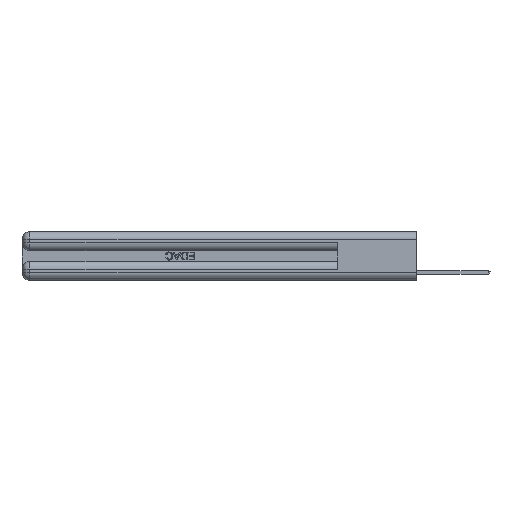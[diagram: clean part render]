
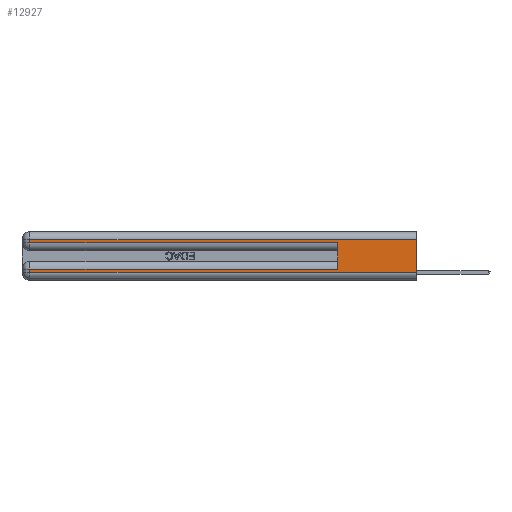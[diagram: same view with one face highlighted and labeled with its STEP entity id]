
A CAD part, left-side view. The second image highlights one B-rep face of the part: STEP entity #12927.
In plain terms, the highlighted planar face has unit normal (-1, 0, 0).
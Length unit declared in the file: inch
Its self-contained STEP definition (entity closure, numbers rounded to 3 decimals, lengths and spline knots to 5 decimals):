
#16 = EDGE_CURVE ( 'NONE', #12384, #17496, #28120, .T. ) ;
#455 = CARTESIAN_POINT ( 'NONE',  ( 0., 2.94, 0.37 ) ) ;
#972 = VECTOR ( 'NONE', #8051, 39.37008 ) ;
#1044 = EDGE_CURVE ( 'NONE', #2760, #12384, #24343, .T. ) ;
#1774 = ORIENTED_EDGE ( 'NONE', *, *, #1044, .T. ) ;
#2023 = CARTESIAN_POINT ( 'NONE',  ( 0., 0.6, 0.285 ) ) ;
#2032 = LINE ( 'NONE', #15748, #14031 ) ;
#2161 = DIRECTION ( 'NONE',  ( 0., 1., 0. ) ) ;
#2760 = VERTEX_POINT ( 'NONE', #16759 ) ;
#3290 = VECTOR ( 'NONE', #7493, 39.37008 ) ;
#3392 = VERTEX_POINT ( 'NONE', #27393 ) ;
#3678 = CARTESIAN_POINT ( 'NONE',  ( 0., 2.94, 0.31 ) ) ;
#3795 = DIRECTION ( 'NONE',  ( 0., -1., 0. ) ) ;
#3897 = CARTESIAN_POINT ( 'NONE',  ( 0., 0.6, 0.085 ) ) ;
#3980 = ORIENTED_EDGE ( 'NONE', *, *, #16, .T. ) ;
#4755 = LINE ( 'NONE', #8476, #15632 ) ;
#5237 = VERTEX_POINT ( 'NONE', #11960 ) ;
#5415 = ORIENTED_EDGE ( 'NONE', *, *, #7825, .T. ) ;
#6302 = LINE ( 'NONE', #26485, #3290 ) ;
#6787 = CARTESIAN_POINT ( 'NONE',  ( 0., 2.94, 0.37 ) ) ;
#7024 = CARTESIAN_POINT ( 'NONE',  ( 0., 2.94, 0.285 ) ) ;
#7116 = CARTESIAN_POINT ( 'NONE',  ( 0., 2.94, 0.085 ) ) ;
#7493 = DIRECTION ( 'NONE',  ( 0., -1., 0. ) ) ;
#7512 = DIRECTION ( 'NONE',  ( 0., 0., -1. ) ) ;
#7825 = EDGE_CURVE ( 'NONE', #3392, #5237, #6302, .T. ) ;
#8051 = DIRECTION ( 'NONE',  ( 0., 0., -1. ) ) ;
#8115 = FACE_OUTER_BOUND ( 'NONE', #29629, .T. ) ;
#8476 = CARTESIAN_POINT ( 'NONE',  ( 0., 0.6, 0.145 ) ) ;
#8689 = EDGE_CURVE ( 'NONE', #21512, #19947, #4755, .T. ) ;
#8894 = EDGE_CURVE ( 'NONE', #2760, #5237, #28492, .T. ) ;
#9956 = DIRECTION ( 'NONE',  ( 0., 0., -1. ) ) ;
#10882 = AXIS2_PLACEMENT_3D ( 'NONE', #14233, #11508, #7512 ) ;
#11327 = EDGE_CURVE ( 'NONE', #21512, #23558, #19867, .T. ) ;
#11508 = DIRECTION ( 'NONE',  ( 1., 0., 0. ) ) ;
#11960 = CARTESIAN_POINT ( 'NONE',  ( 0., 0., 0.06 ) ) ;
#12243 = CARTESIAN_POINT ( 'NONE',  ( 0., 0., 0.31 ) ) ;
#12347 = DIRECTION ( 'NONE',  ( 0., 1., 0. ) ) ;
#12384 = VERTEX_POINT ( 'NONE', #3678 ) ;
#12670 = LINE ( 'NONE', #6787, #17531 ) ;
#12927 = ADVANCED_FACE ( 'NONE', ( #8115 ), #28269, .F. ) ;
#13708 = ORIENTED_EDGE ( 'NONE', *, *, #8894, .F. ) ;
#14031 = VECTOR ( 'NONE', #3795, 39.37008 ) ;
#14233 = CARTESIAN_POINT ( 'NONE',  ( 0., 0., 0.37 ) ) ;
#15047 = ORIENTED_EDGE ( 'NONE', *, *, #20040, .T. ) ;
#15254 = ORIENTED_EDGE ( 'NONE', *, *, #23986, .T. ) ;
#15632 = VECTOR ( 'NONE', #15728, 39.37008 ) ;
#15728 = DIRECTION ( 'NONE',  ( 0., 0., 1. ) ) ;
#15748 = CARTESIAN_POINT ( 'NONE',  ( 0., 0., 0.285 ) ) ;
#16605 = DIRECTION ( 'NONE',  ( 0., 0., -1. ) ) ;
#16759 = CARTESIAN_POINT ( 'NONE',  ( 0., 0., 0.31 ) ) ;
#17496 = VERTEX_POINT ( 'NONE', #7024 ) ;
#17531 = VECTOR ( 'NONE', #16605, 39.37008 ) ;
#19489 = VECTOR ( 'NONE', #2161, 39.37008 ) ;
#19867 = LINE ( 'NONE', #25794, #19489 ) ;
#19947 = VERTEX_POINT ( 'NONE', #2023 ) ;
#20040 = EDGE_CURVE ( 'NONE', #17496, #19947, #2032, .T. ) ;
#20163 = ORIENTED_EDGE ( 'NONE', *, *, #8689, .F. ) ;
#21512 = VERTEX_POINT ( 'NONE', #3897 ) ;
#21730 = ORIENTED_EDGE ( 'NONE', *, *, #11327, .T. ) ;
#22314 = CARTESIAN_POINT ( 'NONE',  ( 0., 0., 0.37 ) ) ;
#23558 = VERTEX_POINT ( 'NONE', #7116 ) ;
#23986 = EDGE_CURVE ( 'NONE', #23558, #3392, #12670, .T. ) ;
#24343 = LINE ( 'NONE', #12243, #29162 ) ;
#25566 = VECTOR ( 'NONE', #9956, 39.37008 ) ;
#25794 = CARTESIAN_POINT ( 'NONE',  ( 0., 0., 0.085 ) ) ;
#26485 = CARTESIAN_POINT ( 'NONE',  ( 0., 0., 0.06 ) ) ;
#27393 = CARTESIAN_POINT ( 'NONE',  ( 0., 2.94, 0.06 ) ) ;
#28120 = LINE ( 'NONE', #455, #25566 ) ;
#28269 = PLANE ( 'NONE',  #10882 ) ;
#28492 = LINE ( 'NONE', #22314, #972 ) ;
#29162 = VECTOR ( 'NONE', #12347, 39.37008 ) ;
#29629 = EDGE_LOOP ( 'NONE', ( #13708, #1774, #3980, #15047, #20163, #21730, #15254, #5415 ) ) ;
